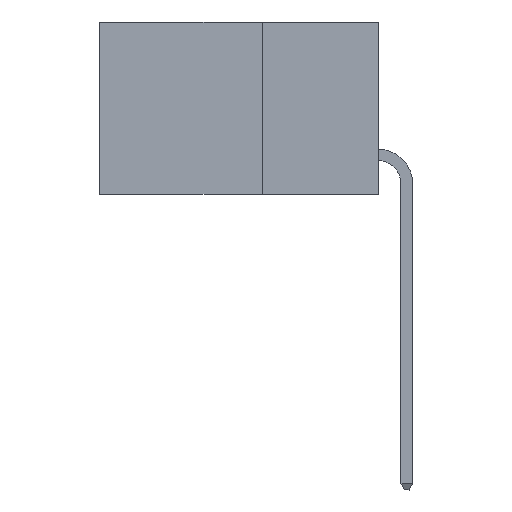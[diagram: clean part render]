
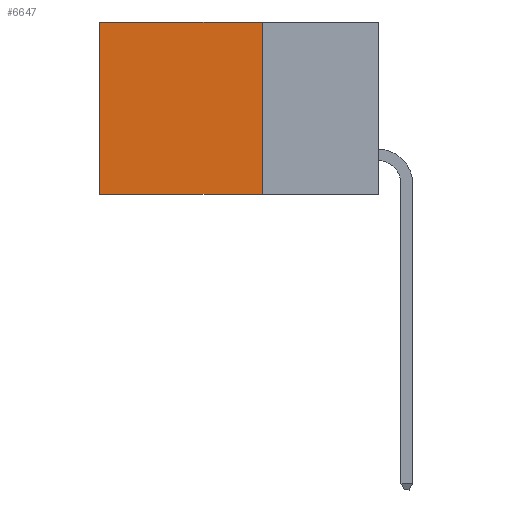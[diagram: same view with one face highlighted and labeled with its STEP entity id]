
A CAD part, left-side view. The second image highlights one B-rep face of the part: STEP entity #6647.
In plain terms, the highlighted planar face has unit normal (-1, 0, 0).
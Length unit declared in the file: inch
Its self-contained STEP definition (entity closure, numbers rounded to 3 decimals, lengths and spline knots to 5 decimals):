
#25 = CARTESIAN_POINT ( 'NONE',  ( 0.2615, 0.25, 0. ) ) ;
#362 = CARTESIAN_POINT ( 'NONE',  ( 0.2615, 0.25, -0.37 ) ) ;
#652 = CARTESIAN_POINT ( 'NONE',  ( 0.2615, 0.6, 0. ) ) ;
#925 = LINE ( 'NONE', #1626, #6318 ) ;
#973 = DIRECTION ( 'NONE',  ( 0., 1., 0. ) ) ;
#1170 = VERTEX_POINT ( 'NONE', #7736 ) ;
#1505 = ORIENTED_EDGE ( 'NONE', *, *, #5712, .F. ) ;
#1626 = CARTESIAN_POINT ( 'NONE',  ( 0.2615, 0.25, -0.37 ) ) ;
#1662 = FACE_OUTER_BOUND ( 'NONE', #3955, .T. ) ;
#2277 = CARTESIAN_POINT ( 'NONE',  ( 0.2615, 0.25, -0.37 ) ) ;
#2339 = AXIS2_PLACEMENT_3D ( 'NONE', #2277, #6798, #7512 ) ;
#2357 = VECTOR ( 'NONE', #4628, 39.37008 ) ;
#2780 = ORIENTED_EDGE ( 'NONE', *, *, #6222, .F. ) ;
#3124 = VECTOR ( 'NONE', #5223, 39.37008 ) ;
#3139 = EDGE_CURVE ( 'NONE', #7756, #4740, #6582, .T. ) ;
#3471 = VERTEX_POINT ( 'NONE', #5757 ) ;
#3955 = EDGE_LOOP ( 'NONE', ( #7158, #2780, #1505, #8768 ) ) ;
#4628 = DIRECTION ( 'NONE',  ( 0., 0., -1. ) ) ;
#4740 = VERTEX_POINT ( 'NONE', #652 ) ;
#5037 = LINE ( 'NONE', #7245, #3124 ) ;
#5104 = DIRECTION ( 'NONE',  ( 0., 1., 0. ) ) ;
#5223 = DIRECTION ( 'NONE',  ( 0., 0., -1. ) ) ;
#5450 = LINE ( 'NONE', #362, #2357 ) ;
#5712 = EDGE_CURVE ( 'NONE', #7756, #3471, #5450, .T. ) ;
#5757 = CARTESIAN_POINT ( 'NONE',  ( 0.2615, 0.25, -0.37 ) ) ;
#6222 = EDGE_CURVE ( 'NONE', #3471, #1170, #925, .T. ) ;
#6318 = VECTOR ( 'NONE', #973, 39.37008 ) ;
#6582 = LINE ( 'NONE', #25, #7722 ) ;
#6647 = ADVANCED_FACE ( 'NONE', ( #1662 ), #8849, .F. ) ;
#6798 = DIRECTION ( 'NONE',  ( 1., 0., 0. ) ) ;
#7158 = ORIENTED_EDGE ( 'NONE', *, *, #8023, .T. ) ;
#7245 = CARTESIAN_POINT ( 'NONE',  ( 0.2615, 0.6, -0.37 ) ) ;
#7512 = DIRECTION ( 'NONE',  ( 0., 0., -1. ) ) ;
#7722 = VECTOR ( 'NONE', #5104, 39.37008 ) ;
#7736 = CARTESIAN_POINT ( 'NONE',  ( 0.2615, 0.6, -0.37 ) ) ;
#7756 = VERTEX_POINT ( 'NONE', #9232 ) ;
#8023 = EDGE_CURVE ( 'NONE', #4740, #1170, #5037, .T. ) ;
#8768 = ORIENTED_EDGE ( 'NONE', *, *, #3139, .T. ) ;
#8849 = PLANE ( 'NONE',  #2339 ) ;
#9232 = CARTESIAN_POINT ( 'NONE',  ( 0.2615, 0.25, 0. ) ) ;
